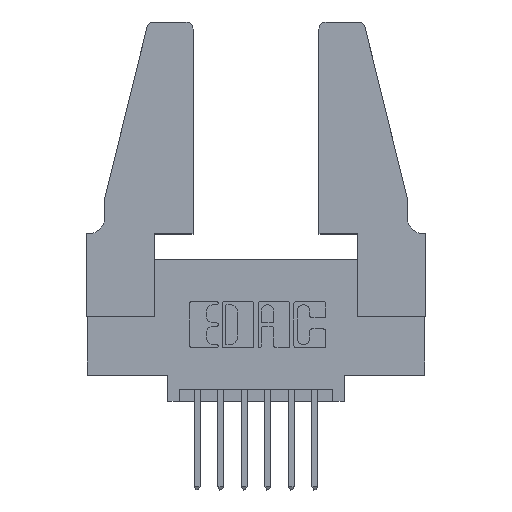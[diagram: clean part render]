
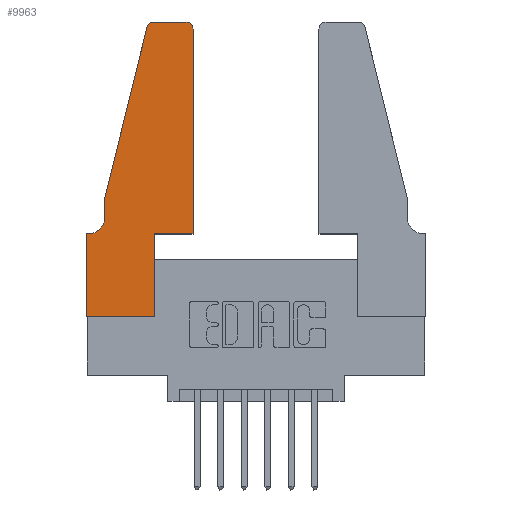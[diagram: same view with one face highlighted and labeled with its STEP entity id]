
A CAD part, top view. The second image highlights one B-rep face of the part: STEP entity #9963.
In plain terms, the highlighted planar face has unit normal (0, 0, 1).
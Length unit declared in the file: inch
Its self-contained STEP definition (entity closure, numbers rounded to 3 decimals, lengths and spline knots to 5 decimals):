
#474 = ORIENTED_EDGE ( 'NONE', *, *, #9602, .T. ) ;
#521 = EDGE_CURVE ( 'NONE', #6074, #2888, #8049, .T. ) ;
#696 = VECTOR ( 'NONE', #6978, 39.37008 ) ;
#907 = CARTESIAN_POINT ( 'NONE',  ( 0.2865, 0.35, 0.37 ) ) ;
#924 = ORIENTED_EDGE ( 'NONE', *, *, #9650, .T. ) ;
#1350 = LINE ( 'NONE', #4436, #6018 ) ;
#1531 = ORIENTED_EDGE ( 'NONE', *, *, #521, .T. ) ;
#1622 = DIRECTION ( 'NONE',  ( -0.239, -0.971, 0. ) ) ;
#1741 = ORIENTED_EDGE ( 'NONE', *, *, #8045, .T. ) ;
#1980 = CARTESIAN_POINT ( 'NONE',  ( 0.0055, 0.42, 0.37 ) ) ;
#2060 = CARTESIAN_POINT ( 'NONE',  ( 0.0755, 0.35, 0.37 ) ) ;
#2086 = CARTESIAN_POINT ( 'NONE',  ( 0.284, 1.22, 0.37 ) ) ;
#2189 = LINE ( 'NONE', #9673, #6830 ) ;
#2543 = VERTEX_POINT ( 'NONE', #11838 ) ;
#2548 = EDGE_LOOP ( 'NONE', ( #5077, #2728, #3616, #11595, #3364, #7079, #3085, #1741, #3753, #924, #474, #1531 ) ) ;
#2562 = DIRECTION ( 'NONE',  ( 0., -1., 0. ) ) ;
#2617 = DIRECTION ( 'NONE',  ( 1., 0., 0. ) ) ;
#2703 = VERTEX_POINT ( 'NONE', #6448 ) ;
#2728 = ORIENTED_EDGE ( 'NONE', *, *, #10151, .T. ) ;
#2888 = VERTEX_POINT ( 'NONE', #9718 ) ;
#2920 = DIRECTION ( 'NONE',  ( -1., 0., 0. ) ) ;
#2988 = CARTESIAN_POINT ( 'NONE',  ( 0.4505, 1.22, 0.37 ) ) ;
#3029 = DIRECTION ( 'NONE',  ( 1., 0., 0. ) ) ;
#3039 = CARTESIAN_POINT ( 'NONE',  ( 0.284, 1.25, 0.37 ) ) ;
#3047 = DIRECTION ( 'NONE',  ( 0., 1., 0. ) ) ;
#3085 = ORIENTED_EDGE ( 'NONE', *, *, #5104, .T. ) ;
#3179 = FACE_OUTER_BOUND ( 'NONE', #2548, .T. ) ;
#3247 = VERTEX_POINT ( 'NONE', #907 ) ;
#3265 = CARTESIAN_POINT ( 'NONE',  ( 0., 0., 0.37 ) ) ;
#3364 = ORIENTED_EDGE ( 'NONE', *, *, #9472, .T. ) ;
#3386 = VERTEX_POINT ( 'NONE', #3039 ) ;
#3484 = LINE ( 'NONE', #3265, #696 ) ;
#3616 = ORIENTED_EDGE ( 'NONE', *, *, #7030, .T. ) ;
#3617 = CIRCLE ( 'NONE', #8747, 0.03 ) ;
#3753 = ORIENTED_EDGE ( 'NONE', *, *, #6446, .T. ) ;
#3862 = CARTESIAN_POINT ( 'NONE',  ( 0., 0.35, 0.37 ) ) ;
#3865 = VECTOR ( 'NONE', #1622, 39.37008 ) ;
#4204 = DIRECTION ( 'NONE',  ( 1., 0., 0. ) ) ;
#4436 = CARTESIAN_POINT ( 'NONE',  ( 0.0755, 0.5, 0.37 ) ) ;
#4620 = DIRECTION ( 'NONE',  ( 0., 0., 1. ) ) ;
#4632 = LINE ( 'NONE', #4635, #9185 ) ;
#4635 = CARTESIAN_POINT ( 'NONE',  ( 0.2605, 1.25, 0.37 ) ) ;
#5077 = ORIENTED_EDGE ( 'NONE', *, *, #11142, .T. ) ;
#5104 = EDGE_CURVE ( 'NONE', #6061, #7811, #3484, .T. ) ;
#5259 = VERTEX_POINT ( 'NONE', #11638 ) ;
#5326 = VECTOR ( 'NONE', #8150, 39.37008 ) ;
#5702 = CARTESIAN_POINT ( 'NONE',  ( 0., 0., 0.37 ) ) ;
#5714 = VERTEX_POINT ( 'NONE', #10692 ) ;
#5800 = VECTOR ( 'NONE', #11339, 39.37008 ) ;
#5927 = CARTESIAN_POINT ( 'NONE',  ( 0.4505, 0.35, 0.37 ) ) ;
#6018 = VECTOR ( 'NONE', #2562, 39.37008 ) ;
#6061 = VERTEX_POINT ( 'NONE', #3862 ) ;
#6064 = VERTEX_POINT ( 'NONE', #8480 ) ;
#6074 = VERTEX_POINT ( 'NONE', #2988 ) ;
#6446 = EDGE_CURVE ( 'NONE', #5714, #3247, #9899, .T. ) ;
#6448 = CARTESIAN_POINT ( 'NONE',  ( 0.25487, 1.22718, 0.37 ) ) ;
#6735 = LINE ( 'NONE', #2060, #9162 ) ;
#6830 = VECTOR ( 'NONE', #4204, 39.37008 ) ;
#6978 = DIRECTION ( 'NONE',  ( 0., -1., 0. ) ) ;
#7030 = EDGE_CURVE ( 'NONE', #2703, #9655, #10847, .T. ) ;
#7031 = EDGE_CURVE ( 'NONE', #9655, #6064, #1350, .T. ) ;
#7079 = ORIENTED_EDGE ( 'NONE', *, *, #7872, .T. ) ;
#7185 = CARTESIAN_POINT ( 'NONE',  ( 0.0755, 0.5, 0.37 ) ) ;
#7246 = CARTESIAN_POINT ( 'NONE',  ( 0.2865, 0.35, 0.37 ) ) ;
#7330 = CARTESIAN_POINT ( 'NONE',  ( 0., 0.35, 0.37 ) ) ;
#7389 = DIRECTION ( 'NONE',  ( -1., 0., 0. ) ) ;
#7699 = CARTESIAN_POINT ( 'NONE',  ( 0.4505, 0.35, 0.37 ) ) ;
#7811 = VERTEX_POINT ( 'NONE', #5702 ) ;
#7872 = EDGE_CURVE ( 'NONE', #5259, #6061, #6735, .T. ) ;
#8045 = EDGE_CURVE ( 'NONE', #7811, #5714, #2189, .T. ) ;
#8049 = CIRCLE ( 'NONE', #11743, 0.03 ) ;
#8150 = DIRECTION ( 'NONE',  ( 0., 1., 0. ) ) ;
#8458 = DIRECTION ( 'NONE',  ( 0., 0., -1. ) ) ;
#8480 = CARTESIAN_POINT ( 'NONE',  ( 0.0755, 0.42, 0.37 ) ) ;
#8520 = LINE ( 'NONE', #5927, #5800 ) ;
#8535 = DIRECTION ( 'NONE',  ( -1., 0., 0. ) ) ;
#8562 = DIRECTION ( 'NONE',  ( 0., 0., 1. ) ) ;
#8690 = CARTESIAN_POINT ( 'NONE',  ( 0.0755, 0.5, 0.37 ) ) ;
#8747 = AXIS2_PLACEMENT_3D ( 'NONE', #2086, #8562, #3029 ) ;
#8803 = VECTOR ( 'NONE', #3047, 39.37008 ) ;
#9162 = VECTOR ( 'NONE', #8535, 39.37008 ) ;
#9185 = VECTOR ( 'NONE', #7389, 39.37008 ) ;
#9366 = LINE ( 'NONE', #7699, #8803 ) ;
#9472 = EDGE_CURVE ( 'NONE', #6064, #5259, #10225, .T. ) ;
#9602 = EDGE_CURVE ( 'NONE', #2543, #6074, #9366, .T. ) ;
#9650 = EDGE_CURVE ( 'NONE', #3247, #2543, #8520, .T. ) ;
#9655 = VERTEX_POINT ( 'NONE', #8690 ) ;
#9673 = CARTESIAN_POINT ( 'NONE',  ( 0., 0., 0.37 ) ) ;
#9718 = CARTESIAN_POINT ( 'NONE',  ( 0.4205, 1.25, 0.37 ) ) ;
#9899 = LINE ( 'NONE', #7246, #5326 ) ;
#9963 = ADVANCED_FACE ( 'NONE', ( #3179 ), #10060, .T. ) ;
#10060 = PLANE ( 'NONE',  #11360 ) ;
#10151 = EDGE_CURVE ( 'NONE', #3386, #2703, #3617, .T. ) ;
#10225 = CIRCLE ( 'NONE', #11785, 0.07 ) ;
#10692 = CARTESIAN_POINT ( 'NONE',  ( 0.2865, 0., 0.37 ) ) ;
#10847 = LINE ( 'NONE', #7185, #3865 ) ;
#10959 = DIRECTION ( 'NONE',  ( 1., 0., 0. ) ) ;
#11131 = CARTESIAN_POINT ( 'NONE',  ( 0.4205, 1.22, 0.37 ) ) ;
#11142 = EDGE_CURVE ( 'NONE', #2888, #3386, #4632, .T. ) ;
#11256 = DIRECTION ( 'NONE',  ( 0., 0., 1. ) ) ;
#11339 = DIRECTION ( 'NONE',  ( 1., 0., 0. ) ) ;
#11360 = AXIS2_PLACEMENT_3D ( 'NONE', #7330, #4620, #10959 ) ;
#11595 = ORIENTED_EDGE ( 'NONE', *, *, #7031, .T. ) ;
#11638 = CARTESIAN_POINT ( 'NONE',  ( 0.0055, 0.35, 0.37 ) ) ;
#11743 = AXIS2_PLACEMENT_3D ( 'NONE', #11131, #11256, #2617 ) ;
#11785 = AXIS2_PLACEMENT_3D ( 'NONE', #1980, #8458, #2920 ) ;
#11838 = CARTESIAN_POINT ( 'NONE',  ( 0.4505, 0.35, 0.37 ) ) ;
